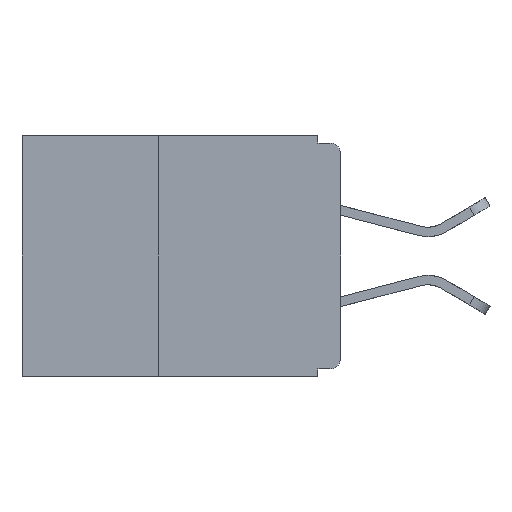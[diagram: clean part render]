
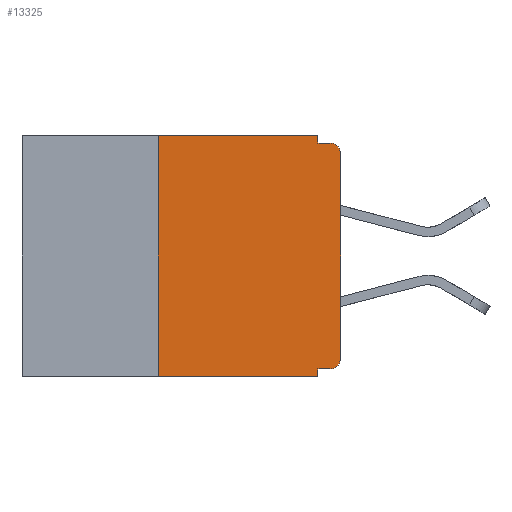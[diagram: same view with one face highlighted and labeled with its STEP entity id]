
A CAD part, left-side view. The second image highlights one B-rep face of the part: STEP entity #13325.
In plain terms, the highlighted planar face has unit normal (-1, 0, 0).
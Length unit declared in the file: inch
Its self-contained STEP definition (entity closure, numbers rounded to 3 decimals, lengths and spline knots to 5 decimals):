
#474 = ORIENTED_EDGE ( 'NONE', *, *, #11149, .F. ) ;
#741 = CARTESIAN_POINT ( 'NONE',  ( 0., 0.015, -0.025 ) ) ;
#1130 = CARTESIAN_POINT ( 'NONE',  ( 0., 0.437, -0.33 ) ) ;
#1224 = DIRECTION ( 'NONE',  ( 0., 0., 1. ) ) ;
#1236 = ORIENTED_EDGE ( 'NONE', *, *, #3725, .T. ) ;
#1300 = PLANE ( 'NONE',  #3841 ) ;
#1630 = ORIENTED_EDGE ( 'NONE', *, *, #5434, .F. ) ;
#1985 = DIRECTION ( 'NONE',  ( 0., 0., -1. ) ) ;
#2028 = DIRECTION ( 'NONE',  ( 0., 0., 1. ) ) ;
#2191 = ORIENTED_EDGE ( 'NONE', *, *, #9719, .T. ) ;
#2210 = CARTESIAN_POINT ( 'NONE',  ( 0., 0.437, 0. ) ) ;
#2423 = VERTEX_POINT ( 'NONE', #7882 ) ;
#2454 = VERTEX_POINT ( 'NONE', #4567 ) ;
#2482 = LINE ( 'NONE', #6832, #11143 ) ;
#2517 = DIRECTION ( 'NONE',  ( 0., 0., -1. ) ) ;
#2743 = FACE_OUTER_BOUND ( 'NONE', #4791, .T. ) ;
#3303 = EDGE_CURVE ( 'NONE', #13960, #2423, #9943, .T. ) ;
#3309 = VECTOR ( 'NONE', #8498, 39.37008 ) ;
#3412 = VERTEX_POINT ( 'NONE', #4792 ) ;
#3725 = EDGE_CURVE ( 'NONE', #5124, #9499, #11027, .T. ) ;
#3841 = AXIS2_PLACEMENT_3D ( 'NONE', #13030, #9573, #2517 ) ;
#4399 = ORIENTED_EDGE ( 'NONE', *, *, #7957, .F. ) ;
#4567 = CARTESIAN_POINT ( 'NONE',  ( 0., 0.031, 0. ) ) ;
#4599 = VECTOR ( 'NONE', #2028, 39.37008 ) ;
#4791 = EDGE_LOOP ( 'NONE', ( #11211, #2191, #12292, #9566, #474, #9941, #1236, #4399, #1630, #11041 ) ) ;
#4792 = CARTESIAN_POINT ( 'NONE',  ( 0., 0.25, 0. ) ) ;
#4842 = VERTEX_POINT ( 'NONE', #12967 ) ;
#5124 = VERTEX_POINT ( 'NONE', #10896 ) ;
#5434 = EDGE_CURVE ( 'NONE', #4842, #10427, #6428, .T. ) ;
#5838 = CARTESIAN_POINT ( 'NONE',  ( 0., 0., -0.025 ) ) ;
#6401 = CARTESIAN_POINT ( 'NONE',  ( 0., 0., -0.01 ) ) ;
#6428 = LINE ( 'NONE', #8524, #3309 ) ;
#6675 = DIRECTION ( 'NONE',  ( 0., -1., 0. ) ) ;
#6741 = LINE ( 'NONE', #8327, #13656 ) ;
#6832 = CARTESIAN_POINT ( 'NONE',  ( 0., 0.031, 0. ) ) ;
#6887 = DIRECTION ( 'NONE',  ( 0., 0., -1. ) ) ;
#7063 = CIRCLE ( 'NONE', #11367, 0.015 ) ;
#7246 = CARTESIAN_POINT ( 'NONE',  ( 0., 0.031, -0.33 ) ) ;
#7523 = VECTOR ( 'NONE', #12329, 39.37008 ) ;
#7604 = VERTEX_POINT ( 'NONE', #11068 ) ;
#7640 = EDGE_CURVE ( 'NONE', #4842, #7604, #7689, .T. ) ;
#7689 = CIRCLE ( 'NONE', #11649, 0.015 ) ;
#7743 = LINE ( 'NONE', #7962, #4599 ) ;
#7882 = CARTESIAN_POINT ( 'NONE',  ( 0., 0.015, -0.01 ) ) ;
#7957 = EDGE_CURVE ( 'NONE', #10427, #9499, #13322, .T. ) ;
#7962 = CARTESIAN_POINT ( 'NONE',  ( 0., 0., 0. ) ) ;
#8138 = DIRECTION ( 'NONE',  ( 0., -1., 0. ) ) ;
#8327 = CARTESIAN_POINT ( 'NONE',  ( 0., 0.25, -0.33 ) ) ;
#8491 = VECTOR ( 'NONE', #8138, 39.37008 ) ;
#8498 = DIRECTION ( 'NONE',  ( 0., 1., 0. ) ) ;
#8524 = CARTESIAN_POINT ( 'NONE',  ( 0., 0., -0.32 ) ) ;
#8944 = EDGE_CURVE ( 'NONE', #2454, #13960, #2482, .T. ) ;
#9018 = DIRECTION ( 'NONE',  ( 0., 0., -1. ) ) ;
#9041 = DIRECTION ( 'NONE',  ( -1., 0., 0. ) ) ;
#9065 = DIRECTION ( 'NONE',  ( -1., 0., 0. ) ) ;
#9068 = CARTESIAN_POINT ( 'NONE',  ( 0., 0.015, -0.305 ) ) ;
#9072 = VERTEX_POINT ( 'NONE', #5838 ) ;
#9499 = VERTEX_POINT ( 'NONE', #7246 ) ;
#9566 = ORIENTED_EDGE ( 'NONE', *, *, #8944, .F. ) ;
#9573 = DIRECTION ( 'NONE',  ( 1., 0., 0. ) ) ;
#9719 = EDGE_CURVE ( 'NONE', #9072, #2423, #7063, .T. ) ;
#9941 = ORIENTED_EDGE ( 'NONE', *, *, #13842, .F. ) ;
#9943 = LINE ( 'NONE', #6401, #12668 ) ;
#10427 = VERTEX_POINT ( 'NONE', #11437 ) ;
#10837 = CARTESIAN_POINT ( 'NONE',  ( 0., 0.031, -0.01 ) ) ;
#10896 = CARTESIAN_POINT ( 'NONE',  ( 0., 0.25, -0.33 ) ) ;
#11027 = LINE ( 'NONE', #1130, #7523 ) ;
#11041 = ORIENTED_EDGE ( 'NONE', *, *, #7640, .T. ) ;
#11068 = CARTESIAN_POINT ( 'NONE',  ( 0., 0., -0.305 ) ) ;
#11143 = VECTOR ( 'NONE', #6887, 39.37008 ) ;
#11149 = EDGE_CURVE ( 'NONE', #3412, #2454, #11619, .T. ) ;
#11211 = ORIENTED_EDGE ( 'NONE', *, *, #11685, .T. ) ;
#11367 = AXIS2_PLACEMENT_3D ( 'NONE', #741, #9041, #1985 ) ;
#11437 = CARTESIAN_POINT ( 'NONE',  ( 0., 0.031, -0.32 ) ) ;
#11619 = LINE ( 'NONE', #2210, #8491 ) ;
#11649 = AXIS2_PLACEMENT_3D ( 'NONE', #9068, #9065, #9018 ) ;
#11685 = EDGE_CURVE ( 'NONE', #7604, #9072, #7743, .T. ) ;
#12215 = CARTESIAN_POINT ( 'NONE',  ( 0., 0.031, -0.33 ) ) ;
#12292 = ORIENTED_EDGE ( 'NONE', *, *, #3303, .F. ) ;
#12329 = DIRECTION ( 'NONE',  ( 0., -1., 0. ) ) ;
#12620 = VECTOR ( 'NONE', #13280, 39.37008 ) ;
#12668 = VECTOR ( 'NONE', #6675, 39.37008 ) ;
#12967 = CARTESIAN_POINT ( 'NONE',  ( 0., 0.015, -0.32 ) ) ;
#13030 = CARTESIAN_POINT ( 'NONE',  ( 0., 0.437, 0. ) ) ;
#13280 = DIRECTION ( 'NONE',  ( 0., 0., -1. ) ) ;
#13322 = LINE ( 'NONE', #12215, #12620 ) ;
#13325 = ADVANCED_FACE ( 'NONE', ( #2743 ), #1300, .F. ) ;
#13656 = VECTOR ( 'NONE', #1224, 39.37008 ) ;
#13842 = EDGE_CURVE ( 'NONE', #5124, #3412, #6741, .T. ) ;
#13960 = VERTEX_POINT ( 'NONE', #10837 ) ;
